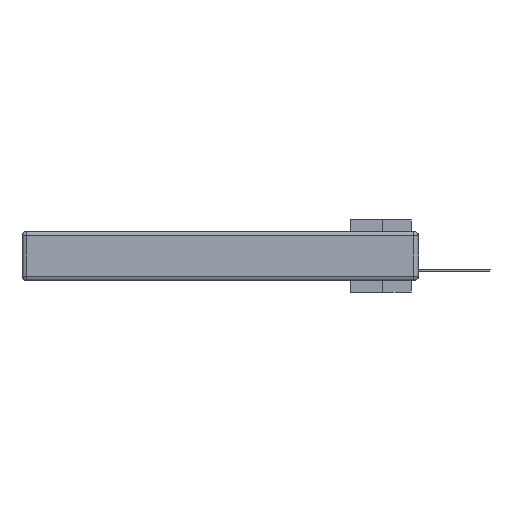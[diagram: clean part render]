
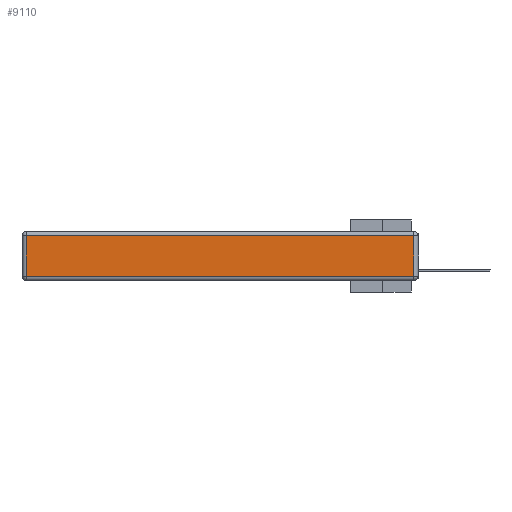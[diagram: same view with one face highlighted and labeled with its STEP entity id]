
A CAD part, left-side view. The second image highlights one B-rep face of the part: STEP entity #9110.
In plain terms, the highlighted planar face has unit normal (-1, 0, 0).
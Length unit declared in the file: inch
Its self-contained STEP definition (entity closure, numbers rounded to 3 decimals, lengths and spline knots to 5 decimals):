
#63 = ORIENTED_EDGE ( 'NONE', *, *, #1588, .T. ) ;
#1588 = EDGE_CURVE ( 'NONE', #21340, #35211, #12779, .T. ) ;
#4766 = CARTESIAN_POINT ( 'NONE',  ( 0., 0.03, -0.313 ) ) ;
#4810 = DIRECTION ( 'NONE',  ( 0., 0., 1. ) ) ;
#9110 = ADVANCED_FACE ( 'NONE', ( #26920 ), #13699, .T. ) ;
#12720 = VECTOR ( 'NONE', #35744, 39.37008 ) ;
#12779 = LINE ( 'NONE', #34537, #25781 ) ;
#13061 = VERTEX_POINT ( 'NONE', #20739 ) ;
#13249 = CARTESIAN_POINT ( 'NONE',  ( 0., 0., -0.313 ) ) ;
#13699 = PLANE ( 'NONE',  #31038 ) ;
#14243 = ORIENTED_EDGE ( 'NONE', *, *, #29382, .T. ) ;
#17341 = DIRECTION ( 'NONE',  ( 0., 1., 0. ) ) ;
#18716 = CARTESIAN_POINT ( 'NONE',  ( 0., 0.03, -0.03 ) ) ;
#19614 = VECTOR ( 'NONE', #20238, 39.37008 ) ;
#20107 = DIRECTION ( 'NONE',  ( -1., 0., 0. ) ) ;
#20238 = DIRECTION ( 'NONE',  ( 0., -1., 0. ) ) ;
#20739 = CARTESIAN_POINT ( 'NONE',  ( 0., 2.72, -0.03 ) ) ;
#21340 = VERTEX_POINT ( 'NONE', #4766 ) ;
#21345 = VERTEX_POINT ( 'NONE', #30023 ) ;
#22062 = EDGE_CURVE ( 'NONE', #13061, #21345, #23069, .T. ) ;
#22144 = VECTOR ( 'NONE', #17341, 39.37008 ) ;
#23069 = LINE ( 'NONE', #38466, #12720 ) ;
#25781 = VECTOR ( 'NONE', #31202, 39.37008 ) ;
#26429 = ORIENTED_EDGE ( 'NONE', *, *, #22062, .T. ) ;
#26920 = FACE_OUTER_BOUND ( 'NONE', #30846, .T. ) ;
#29382 = EDGE_CURVE ( 'NONE', #35211, #13061, #30604, .T. ) ;
#30023 = CARTESIAN_POINT ( 'NONE',  ( 0., 2.72, -0.313 ) ) ;
#30557 = EDGE_CURVE ( 'NONE', #21345, #21340, #36031, .T. ) ;
#30604 = LINE ( 'NONE', #36637, #22144 ) ;
#30846 = EDGE_LOOP ( 'NONE', ( #36460, #63, #14243, #26429 ) ) ;
#31038 = AXIS2_PLACEMENT_3D ( 'NONE', #33183, #20107, #4810 ) ;
#31202 = DIRECTION ( 'NONE',  ( 0., 0., 1. ) ) ;
#33183 = CARTESIAN_POINT ( 'NONE',  ( 0., 0., -0.343 ) ) ;
#34537 = CARTESIAN_POINT ( 'NONE',  ( 0., 0.03, -0.343 ) ) ;
#35211 = VERTEX_POINT ( 'NONE', #18716 ) ;
#35744 = DIRECTION ( 'NONE',  ( 0., 0., -1. ) ) ;
#36031 = LINE ( 'NONE', #13249, #19614 ) ;
#36460 = ORIENTED_EDGE ( 'NONE', *, *, #30557, .T. ) ;
#36637 = CARTESIAN_POINT ( 'NONE',  ( 0., 2.75, -0.03 ) ) ;
#38466 = CARTESIAN_POINT ( 'NONE',  ( 0., 2.72, -0.343 ) ) ;
